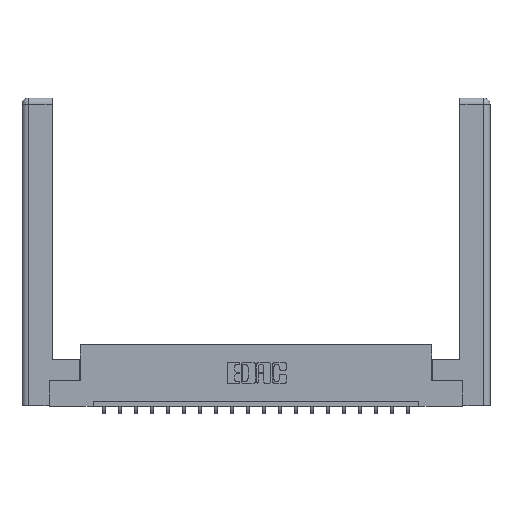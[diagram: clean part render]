
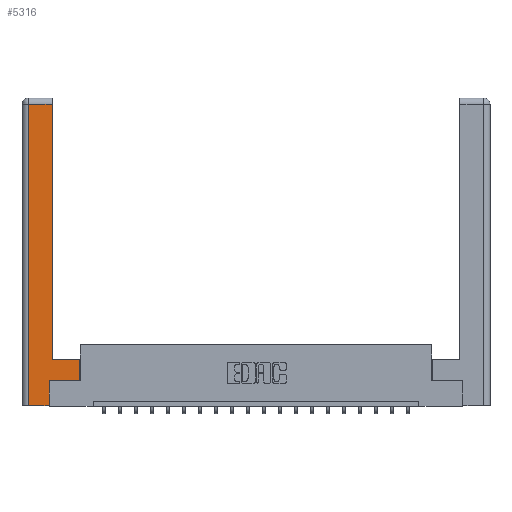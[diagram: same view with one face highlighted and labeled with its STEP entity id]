
A CAD part, top view. The second image highlights one B-rep face of the part: STEP entity #5316.
In plain terms, the highlighted planar face has unit normal (0, 0, 1).
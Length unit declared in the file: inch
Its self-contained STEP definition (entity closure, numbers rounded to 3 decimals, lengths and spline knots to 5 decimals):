
#49 = VERTEX_POINT ( 'NONE', #13314 ) ;
#180 = CARTESIAN_POINT ( 'NONE',  ( 0.265, 0.245, 0. ) ) ;
#546 = DIRECTION ( 'NONE',  ( 1., 0., 0. ) ) ;
#920 = VERTEX_POINT ( 'NONE', #4788 ) ;
#1478 = LINE ( 'NONE', #11293, #2201 ) ;
#1713 = LINE ( 'NONE', #6967, #17258 ) ;
#1853 = DIRECTION ( 'NONE',  ( -1., 0., 0. ) ) ;
#2201 = VECTOR ( 'NONE', #4957, 39.37008 ) ;
#2466 = VECTOR ( 'NONE', #18512, 39.37008 ) ;
#2655 = DIRECTION ( 'NONE',  ( -1., 0., 0. ) ) ;
#2757 = EDGE_CURVE ( 'NONE', #16301, #16853, #12469, .T. ) ;
#3913 = CARTESIAN_POINT ( 'NONE',  ( 0.265, 0., 0. ) ) ;
#4324 = CARTESIAN_POINT ( 'NONE',  ( 0.565, 0.45, 0. ) ) ;
#4704 = ORIENTED_EDGE ( 'NONE', *, *, #10776, .T. ) ;
#4788 = CARTESIAN_POINT ( 'NONE',  ( 0.295, 0.45, 0. ) ) ;
#4957 = DIRECTION ( 'NONE',  ( 0., 1., 0. ) ) ;
#5307 = VECTOR ( 'NONE', #15743, 39.37008 ) ;
#5316 = ADVANCED_FACE ( 'NONE', ( #13830 ), #13988, .F. ) ;
#5381 = CARTESIAN_POINT ( 'NONE',  ( 0.265, 0., 0. ) ) ;
#5791 = CARTESIAN_POINT ( 'NONE',  ( 0.295, 0.45, 0. ) ) ;
#5949 = AXIS2_PLACEMENT_3D ( 'NONE', #20349, #20410, #1853 ) ;
#6236 = CARTESIAN_POINT ( 'NONE',  ( 0.0615, 2.94, 0. ) ) ;
#6967 = CARTESIAN_POINT ( 'NONE',  ( 0.565, 0.245, 0. ) ) ;
#7025 = VECTOR ( 'NONE', #2655, 39.37008 ) ;
#7215 = CARTESIAN_POINT ( 'NONE',  ( 0.565, 0.45, 0. ) ) ;
#7555 = EDGE_CURVE ( 'NONE', #49, #16091, #9323, .T. ) ;
#8570 = ORIENTED_EDGE ( 'NONE', *, *, #20183, .T. ) ;
#8687 = DIRECTION ( 'NONE',  ( 1., 0., 0. ) ) ;
#8790 = CARTESIAN_POINT ( 'NONE',  ( 0.0615, 0., 0. ) ) ;
#9323 = LINE ( 'NONE', #11412, #9824 ) ;
#9824 = VECTOR ( 'NONE', #17486, 39.37008 ) ;
#10120 = ORIENTED_EDGE ( 'NONE', *, *, #11028, .T. ) ;
#10293 = DIRECTION ( 'NONE',  ( 0., -1., 0. ) ) ;
#10688 = CARTESIAN_POINT ( 'NONE',  ( 0.265, 0.245, 0. ) ) ;
#10710 = ORIENTED_EDGE ( 'NONE', *, *, #11127, .T. ) ;
#10776 = EDGE_CURVE ( 'NONE', #16091, #16301, #20314, .T. ) ;
#10924 = LINE ( 'NONE', #5791, #7025 ) ;
#11028 = EDGE_CURVE ( 'NONE', #920, #49, #1478, .T. ) ;
#11127 = EDGE_CURVE ( 'NONE', #15584, #18271, #1713, .T. ) ;
#11293 = CARTESIAN_POINT ( 'NONE',  ( 0.295, 3., 0. ) ) ;
#11412 = CARTESIAN_POINT ( 'NONE',  ( 0.0615, 2.94, 0. ) ) ;
#11906 = VECTOR ( 'NONE', #10293, 39.37008 ) ;
#12469 = LINE ( 'NONE', #3913, #14955 ) ;
#13314 = CARTESIAN_POINT ( 'NONE',  ( 0.295, 2.94, 0. ) ) ;
#13448 = CARTESIAN_POINT ( 'NONE',  ( 0.0615, 0., 0. ) ) ;
#13830 = FACE_OUTER_BOUND ( 'NONE', #16069, .T. ) ;
#13988 = PLANE ( 'NONE',  #5949 ) ;
#14157 = ORIENTED_EDGE ( 'NONE', *, *, #2757, .T. ) ;
#14955 = VECTOR ( 'NONE', #8687, 39.37008 ) ;
#15584 = VERTEX_POINT ( 'NONE', #10688 ) ;
#15743 = DIRECTION ( 'NONE',  ( 0., 1., 0. ) ) ;
#16069 = EDGE_LOOP ( 'NONE', ( #10120, #20333, #4704, #14157, #8570, #10710, #17749, #16588 ) ) ;
#16091 = VERTEX_POINT ( 'NONE', #6236 ) ;
#16301 = VERTEX_POINT ( 'NONE', #13448 ) ;
#16549 = EDGE_CURVE ( 'NONE', #18271, #18993, #19982, .T. ) ;
#16579 = CARTESIAN_POINT ( 'NONE',  ( 0.565, 0.245, 0. ) ) ;
#16588 = ORIENTED_EDGE ( 'NONE', *, *, #18353, .T. ) ;
#16853 = VERTEX_POINT ( 'NONE', #5381 ) ;
#17258 = VECTOR ( 'NONE', #546, 39.37008 ) ;
#17486 = DIRECTION ( 'NONE',  ( -1., 0., 0. ) ) ;
#17749 = ORIENTED_EDGE ( 'NONE', *, *, #16549, .T. ) ;
#17864 = LINE ( 'NONE', #180, #5307 ) ;
#18271 = VERTEX_POINT ( 'NONE', #16579 ) ;
#18353 = EDGE_CURVE ( 'NONE', #18993, #920, #10924, .T. ) ;
#18512 = DIRECTION ( 'NONE',  ( 0., 1., 0. ) ) ;
#18993 = VERTEX_POINT ( 'NONE', #7215 ) ;
#19982 = LINE ( 'NONE', #4324, #2466 ) ;
#20183 = EDGE_CURVE ( 'NONE', #16853, #15584, #17864, .T. ) ;
#20314 = LINE ( 'NONE', #8790, #11906 ) ;
#20333 = ORIENTED_EDGE ( 'NONE', *, *, #7555, .T. ) ;
#20349 = CARTESIAN_POINT ( 'NONE',  ( 0., 0., 0. ) ) ;
#20410 = DIRECTION ( 'NONE',  ( 0., 0., -1. ) ) ;
